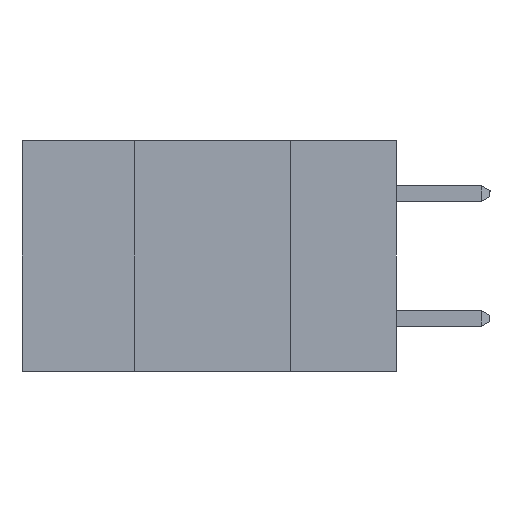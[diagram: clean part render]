
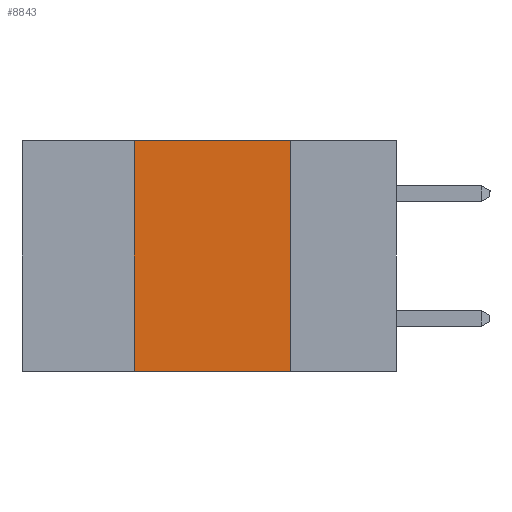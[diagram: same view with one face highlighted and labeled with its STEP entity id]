
A CAD part, left-side view. The second image highlights one B-rep face of the part: STEP entity #8843.
In plain terms, the highlighted planar face has unit normal (-1, 0, 0).
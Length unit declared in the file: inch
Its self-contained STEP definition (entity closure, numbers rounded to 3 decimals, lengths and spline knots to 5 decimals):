
#468 = EDGE_CURVE ( 'NONE', #730, #3069, #1031, .T. ) ;
#563 = CARTESIAN_POINT ( 'NONE',  ( 0., 0.17, -0.37 ) ) ;
#730 = VERTEX_POINT ( 'NONE', #5097 ) ;
#754 = CARTESIAN_POINT ( 'NONE',  ( 0., 0.6, -0.37 ) ) ;
#970 = LINE ( 'NONE', #754, #10407 ) ;
#1031 = LINE ( 'NONE', #2753, #5354 ) ;
#1258 = DIRECTION ( 'NONE',  ( 0., 0., -1. ) ) ;
#1723 = DIRECTION ( 'NONE',  ( 0., -1., 0. ) ) ;
#1780 = CARTESIAN_POINT ( 'NONE',  ( 0., 0.6, 0. ) ) ;
#1832 = ORIENTED_EDGE ( 'NONE', *, *, #1931, .T. ) ;
#1931 = EDGE_CURVE ( 'NONE', #730, #1946, #970, .T. ) ;
#1946 = VERTEX_POINT ( 'NONE', #4167 ) ;
#2120 = FACE_OUTER_BOUND ( 'NONE', #5819, .T. ) ;
#2719 = DIRECTION ( 'NONE',  ( 1., 0., 0. ) ) ;
#2753 = CARTESIAN_POINT ( 'NONE',  ( 0., 0.42, -0.37 ) ) ;
#3069 = VERTEX_POINT ( 'NONE', #8702 ) ;
#3222 = CARTESIAN_POINT ( 'NONE',  ( 0., 0.17, 0. ) ) ;
#3337 = AXIS2_PLACEMENT_3D ( 'NONE', #10181, #2719, #1258 ) ;
#4076 = VERTEX_POINT ( 'NONE', #3222 ) ;
#4167 = CARTESIAN_POINT ( 'NONE',  ( 0., 0.17, -0.37 ) ) ;
#4216 = VECTOR ( 'NONE', #10617, 39.37008 ) ;
#4340 = DIRECTION ( 'NONE',  ( 0., 0., 1. ) ) ;
#5097 = CARTESIAN_POINT ( 'NONE',  ( 0., 0.42, -0.37 ) ) ;
#5354 = VECTOR ( 'NONE', #4340, 39.37008 ) ;
#5753 = DIRECTION ( 'NONE',  ( 0., -1., 0. ) ) ;
#5819 = EDGE_LOOP ( 'NONE', ( #6236, #9096, #8158, #1832 ) ) ;
#6236 = ORIENTED_EDGE ( 'NONE', *, *, #7321, .F. ) ;
#7321 = EDGE_CURVE ( 'NONE', #4076, #1946, #8074, .T. ) ;
#7897 = PLANE ( 'NONE',  #3337 ) ;
#8074 = LINE ( 'NONE', #563, #4216 ) ;
#8158 = ORIENTED_EDGE ( 'NONE', *, *, #468, .F. ) ;
#8387 = EDGE_CURVE ( 'NONE', #3069, #4076, #10047, .T. ) ;
#8702 = CARTESIAN_POINT ( 'NONE',  ( 0., 0.42, 0. ) ) ;
#8843 = ADVANCED_FACE ( 'NONE', ( #2120 ), #7897, .F. ) ;
#9096 = ORIENTED_EDGE ( 'NONE', *, *, #8387, .F. ) ;
#9408 = VECTOR ( 'NONE', #5753, 39.37008 ) ;
#10047 = LINE ( 'NONE', #1780, #9408 ) ;
#10181 = CARTESIAN_POINT ( 'NONE',  ( 0., 0.6, 0. ) ) ;
#10407 = VECTOR ( 'NONE', #1723, 39.37008 ) ;
#10617 = DIRECTION ( 'NONE',  ( 0., 0., -1. ) ) ;
